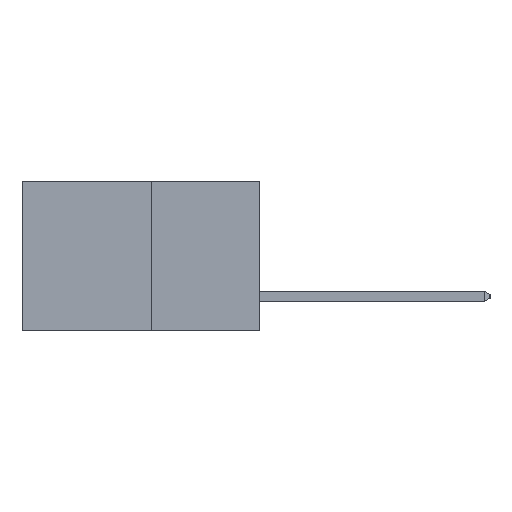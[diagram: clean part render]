
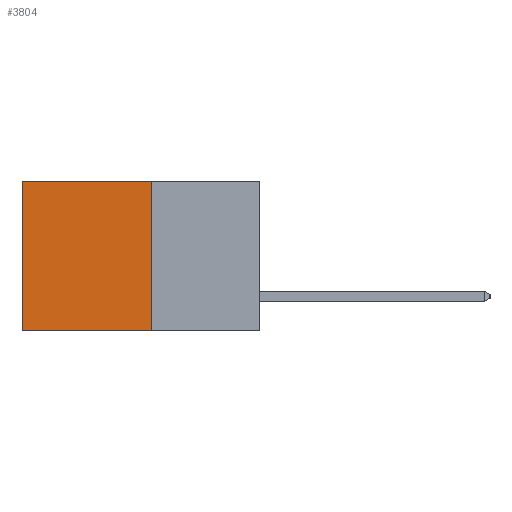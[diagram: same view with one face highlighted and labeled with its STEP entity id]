
A CAD part, left-side view. The second image highlights one B-rep face of the part: STEP entity #3804.
In plain terms, the highlighted planar face has unit normal (-1, 0, 0).
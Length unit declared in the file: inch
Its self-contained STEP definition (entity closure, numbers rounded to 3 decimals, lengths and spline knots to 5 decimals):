
#42 = VECTOR ( 'NONE', #7094, 39.37008 ) ;
#175 = EDGE_CURVE ( 'NONE', #655, #6244, #6935, .T. ) ;
#605 = DIRECTION ( 'NONE',  ( 0., 0., -1. ) ) ;
#655 = VERTEX_POINT ( 'NONE', #5303 ) ;
#681 = EDGE_CURVE ( 'NONE', #6244, #4018, #8154, .T. ) ;
#930 = DIRECTION ( 'NONE',  ( 0., 1., 0. ) ) ;
#1244 = EDGE_LOOP ( 'NONE', ( #7538, #4744, #4612, #8972 ) ) ;
#1958 = CARTESIAN_POINT ( 'NONE',  ( 0.277, 0.59, -0.37 ) ) ;
#2492 = CARTESIAN_POINT ( 'NONE',  ( 0.277, 0.27, -0.37 ) ) ;
#2679 = AXIS2_PLACEMENT_3D ( 'NONE', #2492, #7404, #605 ) ;
#2821 = PLANE ( 'NONE',  #2679 ) ;
#2995 = CARTESIAN_POINT ( 'NONE',  ( 0.277, 0.27, -0.37 ) ) ;
#3166 = LINE ( 'NONE', #7132, #42 ) ;
#3804 = ADVANCED_FACE ( 'NONE', ( #9429 ), #2821, .F. ) ;
#4018 = VERTEX_POINT ( 'NONE', #1958 ) ;
#4097 = CARTESIAN_POINT ( 'NONE',  ( 0.277, 0.59, 0. ) ) ;
#4108 = VECTOR ( 'NONE', #6018, 39.37008 ) ;
#4612 = ORIENTED_EDGE ( 'NONE', *, *, #175, .F. ) ;
#4687 = CARTESIAN_POINT ( 'NONE',  ( 0.277, 0.27, -0.37 ) ) ;
#4744 = ORIENTED_EDGE ( 'NONE', *, *, #681, .F. ) ;
#5182 = VECTOR ( 'NONE', #6054, 39.37008 ) ;
#5287 = CARTESIAN_POINT ( 'NONE',  ( 0.277, 0.27, -0.37 ) ) ;
#5303 = CARTESIAN_POINT ( 'NONE',  ( 0.277, 0.27, 0. ) ) ;
#5825 = EDGE_CURVE ( 'NONE', #655, #6527, #3166, .T. ) ;
#6018 = DIRECTION ( 'NONE',  ( 0., 0., -1. ) ) ;
#6048 = CARTESIAN_POINT ( 'NONE',  ( 0.277, 0.59, -0.37 ) ) ;
#6054 = DIRECTION ( 'NONE',  ( 0., 0., -1. ) ) ;
#6073 = EDGE_CURVE ( 'NONE', #6527, #4018, #6140, .T. ) ;
#6140 = LINE ( 'NONE', #6048, #4108 ) ;
#6231 = VECTOR ( 'NONE', #930, 39.37008 ) ;
#6244 = VERTEX_POINT ( 'NONE', #5287 ) ;
#6527 = VERTEX_POINT ( 'NONE', #4097 ) ;
#6935 = LINE ( 'NONE', #4687, #5182 ) ;
#7094 = DIRECTION ( 'NONE',  ( 0., 1., 0. ) ) ;
#7132 = CARTESIAN_POINT ( 'NONE',  ( 0.277, 0.27, 0. ) ) ;
#7404 = DIRECTION ( 'NONE',  ( 1., 0., 0. ) ) ;
#7538 = ORIENTED_EDGE ( 'NONE', *, *, #6073, .T. ) ;
#8154 = LINE ( 'NONE', #2995, #6231 ) ;
#8972 = ORIENTED_EDGE ( 'NONE', *, *, #5825, .T. ) ;
#9429 = FACE_OUTER_BOUND ( 'NONE', #1244, .T. ) ;
